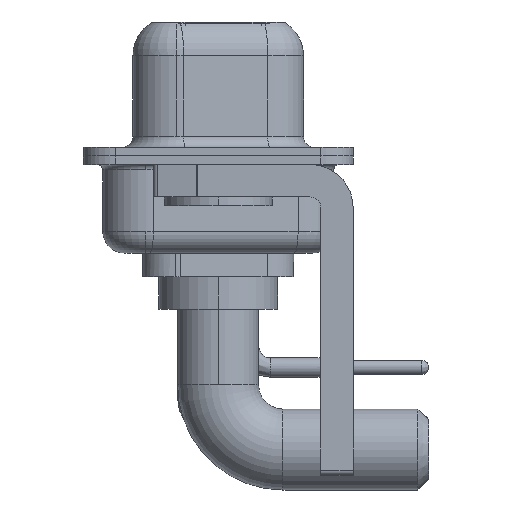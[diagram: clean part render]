
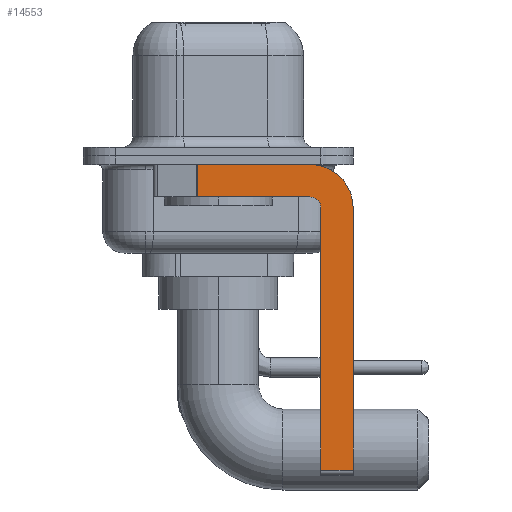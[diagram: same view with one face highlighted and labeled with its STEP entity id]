
A CAD part, left-side view. The second image highlights one B-rep face of the part: STEP entity #14553.
In plain terms, the highlighted planar face has unit normal (-1, 0, 0).
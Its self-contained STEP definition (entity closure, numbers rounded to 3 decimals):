
#267 = AXIS2_PLACEMENT_3D ( 'NONE', #8358, #4682, #4355 ) ;
#318 = EDGE_CURVE ( 'NONE', #4984, #2998, #14168, .T. ) ;
#534 = DIRECTION ( 'NONE',  ( 1., 0., 0. ) ) ;
#548 = CARTESIAN_POINT ( 'NONE',  ( -2.9, -4.25, -1.9 ) ) ;
#726 = ORIENTED_EDGE ( 'NONE', *, *, #4069, .F. ) ;
#871 = CIRCLE ( 'NONE', #267, 0.5 ) ;
#906 = VECTOR ( 'NONE', #7417, 1000. ) ;
#1198 = CARTESIAN_POINT ( 'NONE',  ( -2.9, -4.75, -14.55 ) ) ;
#1272 = CARTESIAN_POINT ( 'NONE',  ( -2.9, -4.25, -14.55 ) ) ;
#1810 = ORIENTED_EDGE ( 'NONE', *, *, #5673, .T. ) ;
#1972 = LINE ( 'NONE', #7599, #906 ) ;
#2271 = CARTESIAN_POINT ( 'NONE',  ( -2.9, -4.25, -1.9 ) ) ;
#2858 = CARTESIAN_POINT ( 'NONE',  ( -2.9, 0.978, -1.9 ) ) ;
#2998 = VERTEX_POINT ( 'NONE', #12365 ) ;
#3313 = LINE ( 'NONE', #548, #15116 ) ;
#3343 = LINE ( 'NONE', #16572, #5413 ) ;
#3410 = CARTESIAN_POINT ( 'NONE',  ( -2.9, -6.25, -14.55 ) ) ;
#3492 = ORIENTED_EDGE ( 'NONE', *, *, #9498, .F. ) ;
#4069 = EDGE_CURVE ( 'NONE', #8958, #4984, #7399, .T. ) ;
#4075 = CARTESIAN_POINT ( 'NONE',  ( -2.9, -4.75, -14.8 ) ) ;
#4355 = DIRECTION ( 'NONE',  ( 0., 0., 1. ) ) ;
#4587 = CARTESIAN_POINT ( 'NONE',  ( -2.9, 0.978, -0.4 ) ) ;
#4682 = DIRECTION ( 'NONE',  ( -1., 0., 0. ) ) ;
#4757 = EDGE_CURVE ( 'NONE', #9293, #9214, #6756, .T. ) ;
#4984 = VERTEX_POINT ( 'NONE', #7095 ) ;
#5413 = VECTOR ( 'NONE', #16315, 1000. ) ;
#5673 = EDGE_CURVE ( 'NONE', #9293, #15334, #14830, .T. ) ;
#5765 = VERTEX_POINT ( 'NONE', #2858 ) ;
#6756 = LINE ( 'NONE', #4075, #11837 ) ;
#7095 = CARTESIAN_POINT ( 'NONE',  ( -2.9, -4.25, -0.4 ) ) ;
#7326 = DIRECTION ( 'NONE',  ( 0., 1., 0. ) ) ;
#7399 = LINE ( 'NONE', #13017, #10616 ) ;
#7417 = DIRECTION ( 'NONE',  ( 0., 0., -1. ) ) ;
#7599 = CARTESIAN_POINT ( 'NONE',  ( -2.9, -6.25, -2.4 ) ) ;
#7894 = DIRECTION ( 'NONE',  ( 0., 0., -1. ) ) ;
#8358 = CARTESIAN_POINT ( 'NONE',  ( -2.9, -4.25, -2.4 ) ) ;
#8736 = AXIS2_PLACEMENT_3D ( 'NONE', #13911, #534, #12660 ) ;
#8958 = VERTEX_POINT ( 'NONE', #4587 ) ;
#9105 = DIRECTION ( 'NONE',  ( 0., -1., 0. ) ) ;
#9214 = VERTEX_POINT ( 'NONE', #16175 ) ;
#9268 = EDGE_LOOP ( 'NONE', ( #726, #12363, #3492, #13088, #13328, #1810, #11925, #10103 ) ) ;
#9293 = VERTEX_POINT ( 'NONE', #1198 ) ;
#9498 = EDGE_CURVE ( 'NONE', #17315, #5765, #3313, .T. ) ;
#9604 = EDGE_CURVE ( 'NONE', #2998, #15334, #1972, .T. ) ;
#9868 = VECTOR ( 'NONE', #9105, 1000. ) ;
#10103 = ORIENTED_EDGE ( 'NONE', *, *, #318, .F. ) ;
#10616 = VECTOR ( 'NONE', #12930, 1000. ) ;
#10661 = CARTESIAN_POINT ( 'NONE',  ( -2.9, -4.25, -2.4 ) ) ;
#11837 = VECTOR ( 'NONE', #14956, 1000. ) ;
#11925 = ORIENTED_EDGE ( 'NONE', *, *, #9604, .F. ) ;
#12363 = ORIENTED_EDGE ( 'NONE', *, *, #17164, .T. ) ;
#12365 = CARTESIAN_POINT ( 'NONE',  ( -2.9, -6.25, -2.4 ) ) ;
#12660 = DIRECTION ( 'NONE',  ( 0., 0., -1. ) ) ;
#12930 = DIRECTION ( 'NONE',  ( 0., -1., 0. ) ) ;
#13017 = CARTESIAN_POINT ( 'NONE',  ( -2.9, 3., -0.4 ) ) ;
#13088 = ORIENTED_EDGE ( 'NONE', *, *, #17065, .F. ) ;
#13249 = PLANE ( 'NONE',  #16655 ) ;
#13328 = ORIENTED_EDGE ( 'NONE', *, *, #4757, .F. ) ;
#13595 = FACE_OUTER_BOUND ( 'NONE', #9268, .T. ) ;
#13911 = CARTESIAN_POINT ( 'NONE',  ( -2.9, -4.25, -2.4 ) ) ;
#14168 = CIRCLE ( 'NONE', #8736, 2. ) ;
#14553 = ADVANCED_FACE ( 'NONE', ( #13595 ), #13249, .F. ) ;
#14830 = LINE ( 'NONE', #1272, #9868 ) ;
#14956 = DIRECTION ( 'NONE',  ( 0., 0., 1. ) ) ;
#15116 = VECTOR ( 'NONE', #7326, 1000. ) ;
#15334 = VERTEX_POINT ( 'NONE', #3410 ) ;
#16175 = CARTESIAN_POINT ( 'NONE',  ( -2.9, -4.75, -2.4 ) ) ;
#16195 = DIRECTION ( 'NONE',  ( 1., 0., 0. ) ) ;
#16315 = DIRECTION ( 'NONE',  ( 0., 0., -1. ) ) ;
#16572 = CARTESIAN_POINT ( 'NONE',  ( -2.9, 0.978, -1.9 ) ) ;
#16655 = AXIS2_PLACEMENT_3D ( 'NONE', #10661, #16195, #7894 ) ;
#17065 = EDGE_CURVE ( 'NONE', #9214, #17315, #871, .T. ) ;
#17164 = EDGE_CURVE ( 'NONE', #8958, #5765, #3343, .T. ) ;
#17315 = VERTEX_POINT ( 'NONE', #2271 ) ;
